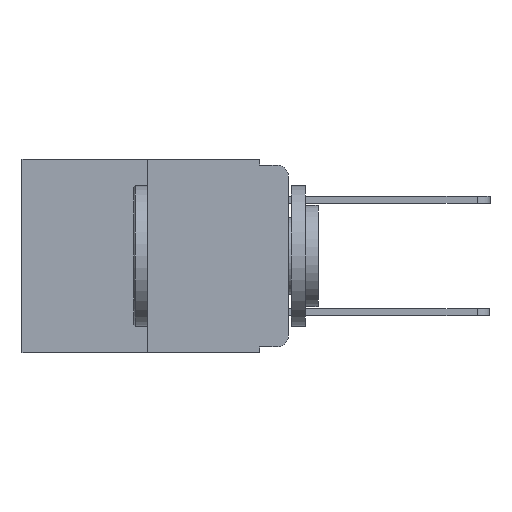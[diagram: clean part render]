
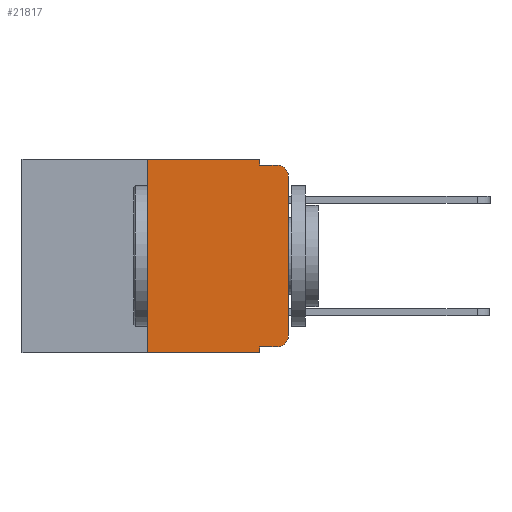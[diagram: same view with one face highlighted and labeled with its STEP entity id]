
A CAD part, left-side view. The second image highlights one B-rep face of the part: STEP entity #21817.
In plain terms, the highlighted planar face has unit normal (-1, 0, 0).
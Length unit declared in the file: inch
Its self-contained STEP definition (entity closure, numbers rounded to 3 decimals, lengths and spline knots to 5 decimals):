
#304 = CIRCLE ( 'NONE', #608, 0.02 ) ;
#509 = PLANE ( 'NONE',  #2074 ) ;
#608 = AXIS2_PLACEMENT_3D ( 'NONE', #9606, #23470, #11593 ) ;
#742 = VECTOR ( 'NONE', #18447, 39.37008 ) ;
#1321 = EDGE_LOOP ( 'NONE', ( #21559, #6331, #12542, #16912, #7635, #25217, #15951, #6719, #15660, #16934 ) ) ;
#1394 = LINE ( 'NONE', #16410, #742 ) ;
#2074 = AXIS2_PLACEMENT_3D ( 'NONE', #24304, #6367, #2628 ) ;
#2467 = VERTEX_POINT ( 'NONE', #13393 ) ;
#2628 = DIRECTION ( 'NONE',  ( 0., 0., -1. ) ) ;
#2693 = AXIS2_PLACEMENT_3D ( 'NONE', #21533, #9593, #23461 ) ;
#3095 = DIRECTION ( 'NONE',  ( 0., 0., -1. ) ) ;
#3247 = CARTESIAN_POINT ( 'NONE',  ( 0., 0.02, -0.333 ) ) ;
#3354 = CARTESIAN_POINT ( 'NONE',  ( 0., 0.02, -0.01 ) ) ;
#3729 = EDGE_CURVE ( 'NONE', #9431, #5654, #19726, .T. ) ;
#3886 = VECTOR ( 'NONE', #15184, 39.37008 ) ;
#5283 = CARTESIAN_POINT ( 'NONE',  ( 0., 0.473, -0.343 ) ) ;
#5335 = LINE ( 'NONE', #8487, #15192 ) ;
#5516 = DIRECTION ( 'NONE',  ( 0., -1., 0. ) ) ;
#5609 = VECTOR ( 'NONE', #24256, 39.37008 ) ;
#5654 = VERTEX_POINT ( 'NONE', #22129 ) ;
#6047 = EDGE_CURVE ( 'NONE', #8619, #9327, #6553, .T. ) ;
#6331 = ORIENTED_EDGE ( 'NONE', *, *, #6047, .T. ) ;
#6367 = DIRECTION ( 'NONE',  ( 1., 0., 0. ) ) ;
#6553 = CIRCLE ( 'NONE', #2693, 0.02 ) ;
#6719 = ORIENTED_EDGE ( 'NONE', *, *, #13500, .F. ) ;
#7262 = EDGE_CURVE ( 'NONE', #18874, #23456, #304, .T. ) ;
#7498 = VECTOR ( 'NONE', #25493, 39.37008 ) ;
#7635 = ORIENTED_EDGE ( 'NONE', *, *, #3729, .F. ) ;
#8373 = EDGE_CURVE ( 'NONE', #5654, #18533, #5335, .T. ) ;
#8487 = CARTESIAN_POINT ( 'NONE',  ( 0., 0.051, 0. ) ) ;
#8619 = VERTEX_POINT ( 'NONE', #19152 ) ;
#9061 = EDGE_CURVE ( 'NONE', #2467, #18874, #11466, .T. ) ;
#9327 = VERTEX_POINT ( 'NONE', #3354 ) ;
#9431 = VERTEX_POINT ( 'NONE', #22105 ) ;
#9437 = VERTEX_POINT ( 'NONE', #10185 ) ;
#9593 = DIRECTION ( 'NONE',  ( -1., 0., 0. ) ) ;
#9606 = CARTESIAN_POINT ( 'NONE',  ( 0., 0.02, -0.313 ) ) ;
#9728 = LINE ( 'NONE', #5283, #3886 ) ;
#9879 = VECTOR ( 'NONE', #23702, 39.37008 ) ;
#10185 = CARTESIAN_POINT ( 'NONE',  ( 0., 0.25, -0.343 ) ) ;
#10219 = CARTESIAN_POINT ( 'NONE',  ( 0., 0.051, -0.01 ) ) ;
#10465 = DIRECTION ( 'NONE',  ( 0., 0., -1. ) ) ;
#10493 = VECTOR ( 'NONE', #3095, 39.37008 ) ;
#11466 = LINE ( 'NONE', #16304, #5609 ) ;
#11593 = DIRECTION ( 'NONE',  ( 0., 0., -1. ) ) ;
#12542 = ORIENTED_EDGE ( 'NONE', *, *, #20532, .F. ) ;
#12902 = CARTESIAN_POINT ( 'NONE',  ( 0., 0.051, 0. ) ) ;
#13118 = EDGE_CURVE ( 'NONE', #23456, #8619, #15114, .T. ) ;
#13393 = CARTESIAN_POINT ( 'NONE',  ( 0., 0.051, -0.333 ) ) ;
#13500 = EDGE_CURVE ( 'NONE', #2467, #19114, #16360, .T. ) ;
#14379 = VECTOR ( 'NONE', #5516, 39.37008 ) ;
#14495 = FACE_OUTER_BOUND ( 'NONE', #1321, .T. ) ;
#15114 = LINE ( 'NONE', #19754, #9879 ) ;
#15184 = DIRECTION ( 'NONE',  ( 0., -1., 0. ) ) ;
#15192 = VECTOR ( 'NONE', #10465, 39.37008 ) ;
#15327 = EDGE_CURVE ( 'NONE', #9437, #9431, #1394, .T. ) ;
#15660 = ORIENTED_EDGE ( 'NONE', *, *, #9061, .T. ) ;
#15951 = ORIENTED_EDGE ( 'NONE', *, *, #19444, .T. ) ;
#16304 = CARTESIAN_POINT ( 'NONE',  ( 0., 0.051, -0.333 ) ) ;
#16360 = LINE ( 'NONE', #12902, #10493 ) ;
#16410 = CARTESIAN_POINT ( 'NONE',  ( 0., 0.25, 0. ) ) ;
#16912 = ORIENTED_EDGE ( 'NONE', *, *, #8373, .F. ) ;
#16934 = ORIENTED_EDGE ( 'NONE', *, *, #7262, .T. ) ;
#18447 = DIRECTION ( 'NONE',  ( 0., 0., 1. ) ) ;
#18533 = VERTEX_POINT ( 'NONE', #10219 ) ;
#18874 = VERTEX_POINT ( 'NONE', #3247 ) ;
#19114 = VERTEX_POINT ( 'NONE', #22030 ) ;
#19152 = CARTESIAN_POINT ( 'NONE',  ( 0., 0., -0.03 ) ) ;
#19444 = EDGE_CURVE ( 'NONE', #9437, #19114, #9728, .T. ) ;
#19562 = CARTESIAN_POINT ( 'NONE',  ( 0., 0.051, -0.01 ) ) ;
#19726 = LINE ( 'NONE', #25176, #14379 ) ;
#19754 = CARTESIAN_POINT ( 'NONE',  ( 0., 0., 0. ) ) ;
#20532 = EDGE_CURVE ( 'NONE', #18533, #9327, #23305, .T. ) ;
#21533 = CARTESIAN_POINT ( 'NONE',  ( 0., 0.02, -0.03 ) ) ;
#21559 = ORIENTED_EDGE ( 'NONE', *, *, #13118, .T. ) ;
#21817 = ADVANCED_FACE ( 'NONE', ( #14495 ), #509, .F. ) ;
#22030 = CARTESIAN_POINT ( 'NONE',  ( 0., 0.051, -0.343 ) ) ;
#22105 = CARTESIAN_POINT ( 'NONE',  ( 0., 0.25, 0. ) ) ;
#22129 = CARTESIAN_POINT ( 'NONE',  ( 0., 0.051, 0. ) ) ;
#22167 = CARTESIAN_POINT ( 'NONE',  ( 0., 0., -0.313 ) ) ;
#23305 = LINE ( 'NONE', #19562, #7498 ) ;
#23456 = VERTEX_POINT ( 'NONE', #22167 ) ;
#23461 = DIRECTION ( 'NONE',  ( 0., 0., -1. ) ) ;
#23470 = DIRECTION ( 'NONE',  ( -1., 0., 0. ) ) ;
#23702 = DIRECTION ( 'NONE',  ( 0., 0., 1. ) ) ;
#24256 = DIRECTION ( 'NONE',  ( 0., -1., 0. ) ) ;
#24304 = CARTESIAN_POINT ( 'NONE',  ( 0., 0.473, 0. ) ) ;
#25176 = CARTESIAN_POINT ( 'NONE',  ( 0., 0.473, 0. ) ) ;
#25217 = ORIENTED_EDGE ( 'NONE', *, *, #15327, .F. ) ;
#25493 = DIRECTION ( 'NONE',  ( 0., -1., 0. ) ) ;
